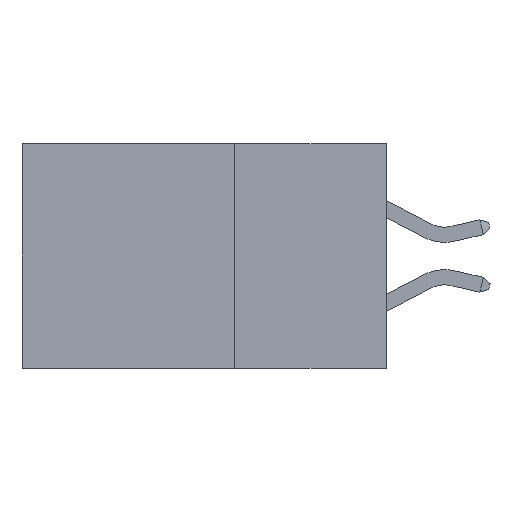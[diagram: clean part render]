
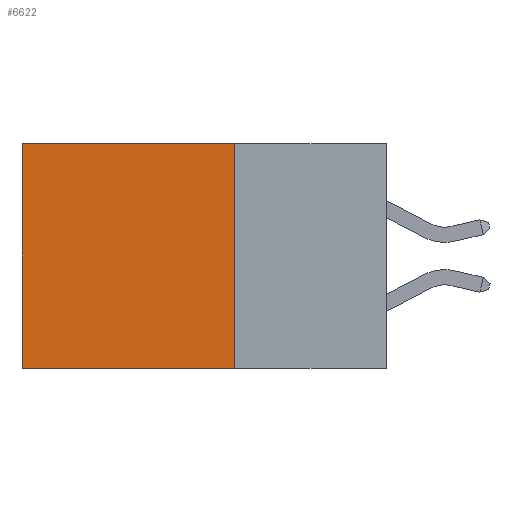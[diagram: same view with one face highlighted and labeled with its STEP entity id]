
A CAD part, left-side view. The second image highlights one B-rep face of the part: STEP entity #6622.
In plain terms, the highlighted planar face has unit normal (-1, 0, 0).
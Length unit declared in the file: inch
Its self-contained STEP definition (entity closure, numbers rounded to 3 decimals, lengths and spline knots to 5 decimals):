
#216 = VERTEX_POINT ( 'NONE', #9721 ) ;
#316 = CARTESIAN_POINT ( 'NONE',  ( 0.298, 0.25, -0.37 ) ) ;
#392 = VECTOR ( 'NONE', #3334, 39.37008 ) ;
#432 = DIRECTION ( 'NONE',  ( 1., 0., 0. ) ) ;
#439 = ORIENTED_EDGE ( 'NONE', *, *, #10273, .T. ) ;
#843 = CARTESIAN_POINT ( 'NONE',  ( 0.298, 0.25, 0. ) ) ;
#1670 = PLANE ( 'NONE',  #6506 ) ;
#1739 = ORIENTED_EDGE ( 'NONE', *, *, #10900, .T. ) ;
#1916 = CARTESIAN_POINT ( 'NONE',  ( 0.298, 0.6, 0. ) ) ;
#2456 = CARTESIAN_POINT ( 'NONE',  ( 0.298, 0.25, 0. ) ) ;
#3277 = ORIENTED_EDGE ( 'NONE', *, *, #3278, .F. ) ;
#3278 = EDGE_CURVE ( 'NONE', #7576, #216, #4478, .T. ) ;
#3334 = DIRECTION ( 'NONE',  ( 0., 0., -1. ) ) ;
#3381 = ORIENTED_EDGE ( 'NONE', *, *, #10292, .F. ) ;
#3389 = VERTEX_POINT ( 'NONE', #1916 ) ;
#4176 = VERTEX_POINT ( 'NONE', #10826 ) ;
#4478 = LINE ( 'NONE', #316, #9764 ) ;
#4897 = DIRECTION ( 'NONE',  ( 0., 1., 0. ) ) ;
#5637 = DIRECTION ( 'NONE',  ( 0., 1., 0. ) ) ;
#5823 = CARTESIAN_POINT ( 'NONE',  ( 0.298, 0.25, -0.37 ) ) ;
#5867 = FACE_OUTER_BOUND ( 'NONE', #10539, .T. ) ;
#6506 = AXIS2_PLACEMENT_3D ( 'NONE', #2456, #432, #11483 ) ;
#6622 = ADVANCED_FACE ( 'NONE', ( #5867 ), #1670, .F. ) ;
#6957 = CARTESIAN_POINT ( 'NONE',  ( 0.298, 0.6, 0. ) ) ;
#7451 = CARTESIAN_POINT ( 'NONE',  ( 0.298, 0.25, 0. ) ) ;
#7576 = VERTEX_POINT ( 'NONE', #5823 ) ;
#7722 = VECTOR ( 'NONE', #9329, 39.37008 ) ;
#9306 = LINE ( 'NONE', #7451, #11788 ) ;
#9329 = DIRECTION ( 'NONE',  ( 0., 0., -1. ) ) ;
#9721 = CARTESIAN_POINT ( 'NONE',  ( 0.298, 0.6, -0.37 ) ) ;
#9764 = VECTOR ( 'NONE', #4897, 39.37008 ) ;
#10273 = EDGE_CURVE ( 'NONE', #4176, #3389, #9306, .T. ) ;
#10292 = EDGE_CURVE ( 'NONE', #4176, #7576, #11207, .T. ) ;
#10353 = LINE ( 'NONE', #6957, #392 ) ;
#10539 = EDGE_LOOP ( 'NONE', ( #1739, #3277, #3381, #439 ) ) ;
#10826 = CARTESIAN_POINT ( 'NONE',  ( 0.298, 0.25, 0. ) ) ;
#10900 = EDGE_CURVE ( 'NONE', #3389, #216, #10353, .T. ) ;
#11207 = LINE ( 'NONE', #843, #7722 ) ;
#11483 = DIRECTION ( 'NONE',  ( 0., 0., -1. ) ) ;
#11788 = VECTOR ( 'NONE', #5637, 39.37008 ) ;
